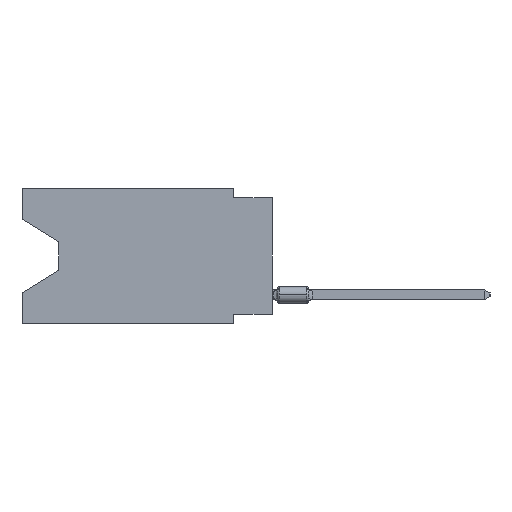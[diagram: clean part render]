
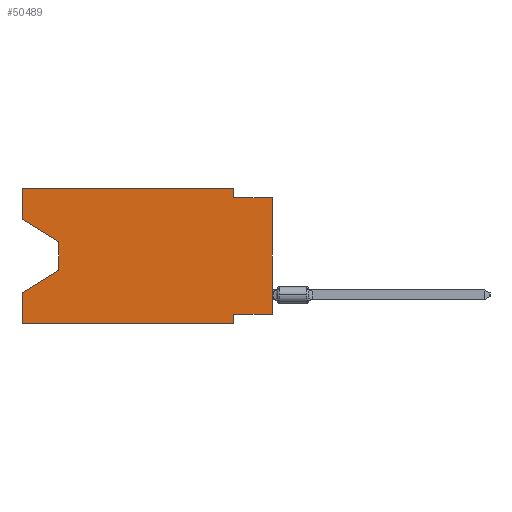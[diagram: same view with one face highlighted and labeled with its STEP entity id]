
A CAD part, left-side view. The second image highlights one B-rep face of the part: STEP entity #50489.
In plain terms, the highlighted planar face has unit normal (-1, 0, 0).
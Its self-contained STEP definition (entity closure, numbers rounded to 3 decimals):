
#684 = DIRECTION ( 'NONE',  ( 0., 0., -1. ) ) ;
#758 = VECTOR ( 'NONE', #33038, 1000. ) ;
#825 = DIRECTION ( 'NONE',  ( 0., 0., -1. ) ) ;
#831 = LINE ( 'NONE', #66284, #61069 ) ;
#2323 = CARTESIAN_POINT ( 'NONE',  ( 0., 16.383, -2.038 ) ) ;
#2327 = CARTESIAN_POINT ( 'NONE',  ( 0., 0., 0. ) ) ;
#3053 = DIRECTION ( 'NONE',  ( 0., -1., 0. ) ) ;
#4144 = CARTESIAN_POINT ( 'NONE',  ( 0., 2.54, -0.635 ) ) ;
#5919 = ORIENTED_EDGE ( 'NONE', *, *, #26078, .T. ) ;
#5988 = VERTEX_POINT ( 'NONE', #66093 ) ;
#6780 = VERTEX_POINT ( 'NONE', #14453 ) ;
#7191 = ORIENTED_EDGE ( 'NONE', *, *, #68140, .F. ) ;
#7340 = DIRECTION ( 'NONE',  ( 0., -0.855, -0.519 ) ) ;
#7688 = VERTEX_POINT ( 'NONE', #4144 ) ;
#10540 = CARTESIAN_POINT ( 'NONE',  ( 0., 16.383, -8.89 ) ) ;
#11676 = DIRECTION ( 'NONE',  ( 0., 0., -1. ) ) ;
#11773 = DIRECTION ( 'NONE',  ( 1., 0., 0. ) ) ;
#12992 = VERTEX_POINT ( 'NONE', #49166 ) ;
#13395 = ORIENTED_EDGE ( 'NONE', *, *, #17513, .F. ) ;
#13769 = VERTEX_POINT ( 'NONE', #16367 ) ;
#14453 = CARTESIAN_POINT ( 'NONE',  ( 0., 2.54, -8.255 ) ) ;
#14477 = CARTESIAN_POINT ( 'NONE',  ( 0., 16.383, 0. ) ) ;
#14734 = EDGE_CURVE ( 'NONE', #58546, #5988, #29287, .T. ) ;
#15901 = LINE ( 'NONE', #10540, #758 ) ;
#16367 = CARTESIAN_POINT ( 'NONE',  ( 0., 16.383, -6.852 ) ) ;
#17043 = LINE ( 'NONE', #38828, #46266 ) ;
#17513 = EDGE_CURVE ( 'NONE', #65623, #7688, #56266, .T. ) ;
#17693 = EDGE_CURVE ( 'NONE', #5988, #13769, #68446, .T. ) ;
#19154 = DIRECTION ( 'NONE',  ( 0., 0., 1. ) ) ;
#19443 = DIRECTION ( 'NONE',  ( 0., 0.855, -0.519 ) ) ;
#19519 = VERTEX_POINT ( 'NONE', #33226 ) ;
#21785 = CARTESIAN_POINT ( 'NONE',  ( 0., 16.383, 0. ) ) ;
#22455 = VECTOR ( 'NONE', #68395, 1000. ) ;
#23804 = ORIENTED_EDGE ( 'NONE', *, *, #24959, .F. ) ;
#24480 = LINE ( 'NONE', #2323, #36712 ) ;
#24780 = VECTOR ( 'NONE', #40164, 1000. ) ;
#24959 = EDGE_CURVE ( 'NONE', #12992, #13769, #68154, .T. ) ;
#26078 = EDGE_CURVE ( 'NONE', #30039, #58546, #24480, .T. ) ;
#27423 = EDGE_LOOP ( 'NONE', ( #5919, #38916, #43870, #23804, #29855, #7191, #64257, #39083, #36472, #13395, #47709, #46560 ) ) ;
#29287 = LINE ( 'NONE', #38342, #69492 ) ;
#29855 = ORIENTED_EDGE ( 'NONE', *, *, #32653, .T. ) ;
#30039 = VERTEX_POINT ( 'NONE', #60953 ) ;
#30335 = CARTESIAN_POINT ( 'NONE',  ( 0., 16.383, 0. ) ) ;
#30468 = VECTOR ( 'NONE', #19443, 1000. ) ;
#30849 = CARTESIAN_POINT ( 'NONE',  ( 0., 13.97, -5.385 ) ) ;
#32653 = EDGE_CURVE ( 'NONE', #12992, #46038, #15901, .T. ) ;
#32818 = CARTESIAN_POINT ( 'NONE',  ( 0., 0., -8.255 ) ) ;
#33038 = DIRECTION ( 'NONE',  ( 0., -1., 0. ) ) ;
#33226 = CARTESIAN_POINT ( 'NONE',  ( 0., 16.383, 0. ) ) ;
#33767 = VECTOR ( 'NONE', #3053, 1000. ) ;
#35989 = EDGE_CURVE ( 'NONE', #19519, #65623, #36400, .T. ) ;
#36400 = LINE ( 'NONE', #30335, #43500 ) ;
#36472 = ORIENTED_EDGE ( 'NONE', *, *, #67068, .F. ) ;
#36712 = VECTOR ( 'NONE', #7340, 1000. ) ;
#38342 = CARTESIAN_POINT ( 'NONE',  ( 0., 13.97, -3.505 ) ) ;
#38828 = CARTESIAN_POINT ( 'NONE',  ( 0., 2.54, -8.89 ) ) ;
#38872 = CARTESIAN_POINT ( 'NONE',  ( 0., 2.54, 0. ) ) ;
#38916 = ORIENTED_EDGE ( 'NONE', *, *, #14734, .T. ) ;
#39083 = ORIENTED_EDGE ( 'NONE', *, *, #57087, .T. ) ;
#39945 = VERTEX_POINT ( 'NONE', #46602 ) ;
#40164 = DIRECTION ( 'NONE',  ( 0., 0., -1. ) ) ;
#40464 = CARTESIAN_POINT ( 'NONE',  ( 0., 16.383, 0. ) ) ;
#40553 = DIRECTION ( 'NONE',  ( 0., 0., 1. ) ) ;
#41448 = EDGE_CURVE ( 'NONE', #30039, #19519, #68738, .T. ) ;
#43500 = VECTOR ( 'NONE', #58245, 1000. ) ;
#43870 = ORIENTED_EDGE ( 'NONE', *, *, #17693, .T. ) ;
#44481 = VECTOR ( 'NONE', #40553, 1000. ) ;
#45426 = CARTESIAN_POINT ( 'NONE',  ( 0., 13.97, -3.505 ) ) ;
#46038 = VERTEX_POINT ( 'NONE', #60476 ) ;
#46089 = DIRECTION ( 'NONE',  ( 0., 1., 0. ) ) ;
#46266 = VECTOR ( 'NONE', #11676, 1000. ) ;
#46560 = ORIENTED_EDGE ( 'NONE', *, *, #41448, .F. ) ;
#46602 = CARTESIAN_POINT ( 'NONE',  ( 0., 0., -0.635 ) ) ;
#47709 = ORIENTED_EDGE ( 'NONE', *, *, #35989, .F. ) ;
#49166 = CARTESIAN_POINT ( 'NONE',  ( 0., 16.383, -8.89 ) ) ;
#50489 = ADVANCED_FACE ( 'NONE', ( #52064 ), #58164, .F. ) ;
#51996 = LINE ( 'NONE', #62768, #33767 ) ;
#52064 = FACE_OUTER_BOUND ( 'NONE', #27423, .T. ) ;
#56266 = LINE ( 'NONE', #68091, #24780 ) ;
#57087 = EDGE_CURVE ( 'NONE', #66317, #39945, #68482, .T. ) ;
#58164 = PLANE ( 'NONE',  #63813 ) ;
#58245 = DIRECTION ( 'NONE',  ( 0., -1., 0. ) ) ;
#58348 = VECTOR ( 'NONE', #19154, 1000. ) ;
#58546 = VERTEX_POINT ( 'NONE', #45426 ) ;
#60476 = CARTESIAN_POINT ( 'NONE',  ( 0., 2.54, -8.89 ) ) ;
#60953 = CARTESIAN_POINT ( 'NONE',  ( 0., 16.383, -2.038 ) ) ;
#61069 = VECTOR ( 'NONE', #46089, 1000. ) ;
#61363 = EDGE_CURVE ( 'NONE', #66317, #6780, #831, .T. ) ;
#62768 = CARTESIAN_POINT ( 'NONE',  ( 0., 0., -0.635 ) ) ;
#63813 = AXIS2_PLACEMENT_3D ( 'NONE', #21785, #11773, #684 ) ;
#64257 = ORIENTED_EDGE ( 'NONE', *, *, #61363, .F. ) ;
#65623 = VERTEX_POINT ( 'NONE', #38872 ) ;
#66093 = CARTESIAN_POINT ( 'NONE',  ( 0., 13.97, -5.385 ) ) ;
#66284 = CARTESIAN_POINT ( 'NONE',  ( 0., 0., -8.255 ) ) ;
#66317 = VERTEX_POINT ( 'NONE', #32818 ) ;
#67068 = EDGE_CURVE ( 'NONE', #7688, #39945, #51996, .T. ) ;
#68091 = CARTESIAN_POINT ( 'NONE',  ( 0., 2.54, 0. ) ) ;
#68140 = EDGE_CURVE ( 'NONE', #6780, #46038, #17043, .T. ) ;
#68154 = LINE ( 'NONE', #14477, #58348 ) ;
#68395 = DIRECTION ( 'NONE',  ( 0., 0., 1. ) ) ;
#68446 = LINE ( 'NONE', #30849, #30468 ) ;
#68482 = LINE ( 'NONE', #2327, #44481 ) ;
#68738 = LINE ( 'NONE', #40464, #22455 ) ;
#69492 = VECTOR ( 'NONE', #825, 1000. ) ;
